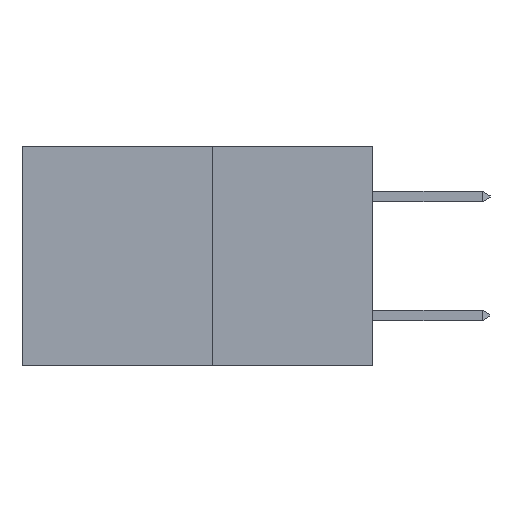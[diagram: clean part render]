
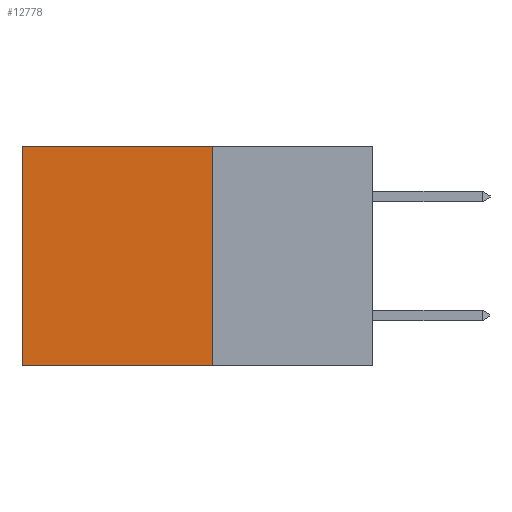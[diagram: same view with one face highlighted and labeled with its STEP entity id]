
A CAD part, left-side view. The second image highlights one B-rep face of the part: STEP entity #12778.
In plain terms, the highlighted planar face has unit normal (-1, 0, 0).
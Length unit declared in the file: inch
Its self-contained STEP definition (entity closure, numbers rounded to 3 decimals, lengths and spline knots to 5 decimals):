
#496 = EDGE_LOOP ( 'NONE', ( #20865, #7973, #8476, #12925 ) ) ;
#696 = CARTESIAN_POINT ( 'NONE',  ( 0.277, 0.59, -0.37 ) ) ;
#733 = DIRECTION ( 'NONE',  ( 0., 0., -1. ) ) ;
#1358 = FACE_OUTER_BOUND ( 'NONE', #496, .T. ) ;
#1495 = VERTEX_POINT ( 'NONE', #696 ) ;
#1669 = CARTESIAN_POINT ( 'NONE',  ( 0.277, 0.27, -0.37 ) ) ;
#2966 = EDGE_CURVE ( 'NONE', #12157, #12782, #18578, .T. ) ;
#4698 = VERTEX_POINT ( 'NONE', #10901 ) ;
#4950 = LINE ( 'NONE', #6753, #5495 ) ;
#5207 = DIRECTION ( 'NONE',  ( 1., 0., 0. ) ) ;
#5495 = VECTOR ( 'NONE', #10000, 39.37008 ) ;
#6050 = CARTESIAN_POINT ( 'NONE',  ( 0.277, 0.27, 0. ) ) ;
#6753 = CARTESIAN_POINT ( 'NONE',  ( 0.277, 0.27, -0.37 ) ) ;
#7509 = LINE ( 'NONE', #21149, #19850 ) ;
#7973 = ORIENTED_EDGE ( 'NONE', *, *, #13610, .F. ) ;
#8476 = ORIENTED_EDGE ( 'NONE', *, *, #2966, .F. ) ;
#9931 = CARTESIAN_POINT ( 'NONE',  ( 0.277, 0.27, 0. ) ) ;
#10000 = DIRECTION ( 'NONE',  ( 0., 1., 0. ) ) ;
#10649 = VECTOR ( 'NONE', #18035, 39.37008 ) ;
#10901 = CARTESIAN_POINT ( 'NONE',  ( 0.277, 0.59, 0. ) ) ;
#11845 = PLANE ( 'NONE',  #12757 ) ;
#12157 = VERTEX_POINT ( 'NONE', #9931 ) ;
#12757 = AXIS2_PLACEMENT_3D ( 'NONE', #15299, #5207, #17027 ) ;
#12778 = ADVANCED_FACE ( 'NONE', ( #1358 ), #11845, .F. ) ;
#12782 = VERTEX_POINT ( 'NONE', #1669 ) ;
#12820 = DIRECTION ( 'NONE',  ( 0., 1., 0. ) ) ;
#12925 = ORIENTED_EDGE ( 'NONE', *, *, #16162, .T. ) ;
#13610 = EDGE_CURVE ( 'NONE', #12782, #1495, #4950, .T. ) ;
#14148 = CARTESIAN_POINT ( 'NONE',  ( 0.277, 0.27, -0.37 ) ) ;
#15299 = CARTESIAN_POINT ( 'NONE',  ( 0.277, 0.27, -0.37 ) ) ;
#15659 = VECTOR ( 'NONE', #12820, 39.37008 ) ;
#16162 = EDGE_CURVE ( 'NONE', #12157, #4698, #20689, .T. ) ;
#17027 = DIRECTION ( 'NONE',  ( 0., 0., -1. ) ) ;
#17362 = EDGE_CURVE ( 'NONE', #4698, #1495, #7509, .T. ) ;
#18035 = DIRECTION ( 'NONE',  ( 0., 0., -1. ) ) ;
#18578 = LINE ( 'NONE', #14148, #10649 ) ;
#19850 = VECTOR ( 'NONE', #733, 39.37008 ) ;
#20689 = LINE ( 'NONE', #6050, #15659 ) ;
#20865 = ORIENTED_EDGE ( 'NONE', *, *, #17362, .T. ) ;
#21149 = CARTESIAN_POINT ( 'NONE',  ( 0.277, 0.59, -0.37 ) ) ;
